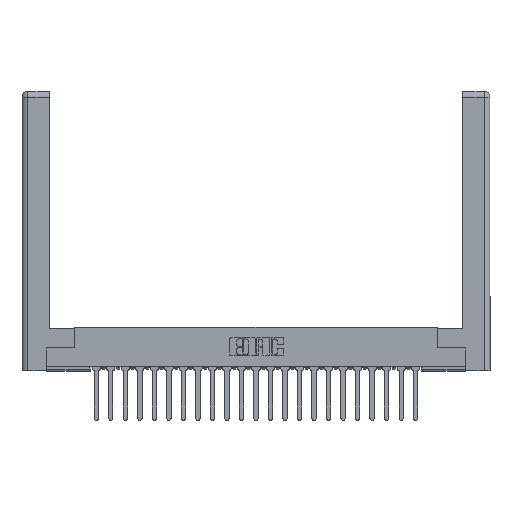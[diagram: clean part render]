
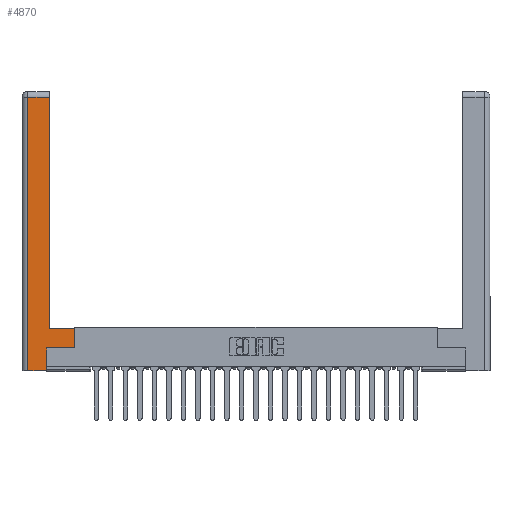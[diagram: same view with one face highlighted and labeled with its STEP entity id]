
A CAD part, top view. The second image highlights one B-rep face of the part: STEP entity #4870.
In plain terms, the highlighted planar face has unit normal (0, 0, 1).
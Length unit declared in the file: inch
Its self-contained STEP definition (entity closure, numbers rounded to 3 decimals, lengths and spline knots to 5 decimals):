
#6 = DIRECTION ( 'NONE',  ( 0., 1., 0. ) ) ;
#18 = EDGE_CURVE ( 'NONE', #4970, #5522, #1642, .T. ) ;
#577 = LINE ( 'NONE', #17559, #17094 ) ;
#739 = ORIENTED_EDGE ( 'NONE', *, *, #7062, .T. ) ;
#1168 = DIRECTION ( 'NONE',  ( 0., 0., -1. ) ) ;
#1177 = EDGE_CURVE ( 'NONE', #13833, #18348, #10896, .T. ) ;
#1642 = LINE ( 'NONE', #16851, #24171 ) ;
#1664 = DIRECTION ( 'NONE',  ( -1., 0., 0. ) ) ;
#2560 = EDGE_LOOP ( 'NONE', ( #3241, #9305, #17655, #739, #11428, #19648, #7668, #17305 ) ) ;
#3241 = ORIENTED_EDGE ( 'NONE', *, *, #19728, .T. ) ;
#3547 = PLANE ( 'NONE',  #6704 ) ;
#4024 = CARTESIAN_POINT ( 'NONE',  ( 0.0615, 2.94, 0. ) ) ;
#4086 = VECTOR ( 'NONE', #6, 39.37008 ) ;
#4566 = CARTESIAN_POINT ( 'NONE',  ( 0.295, 2.94, 0. ) ) ;
#4767 = EDGE_CURVE ( 'NONE', #21797, #19455, #18626, .T. ) ;
#4870 = ADVANCED_FACE ( 'NONE', ( #11147 ), #3547, .F. ) ;
#4970 = VERTEX_POINT ( 'NONE', #4024 ) ;
#5487 = CARTESIAN_POINT ( 'NONE',  ( 0.265, 0., 0. ) ) ;
#5522 = VERTEX_POINT ( 'NONE', #14090 ) ;
#5541 = VECTOR ( 'NONE', #15188, 39.37008 ) ;
#6074 = CARTESIAN_POINT ( 'NONE',  ( 0.0615, 2.94, 0. ) ) ;
#6196 = DIRECTION ( 'NONE',  ( -1., 0., 0. ) ) ;
#6300 = DIRECTION ( 'NONE',  ( 0., 1., 0. ) ) ;
#6704 = AXIS2_PLACEMENT_3D ( 'NONE', #16386, #1168, #1664 ) ;
#7062 = EDGE_CURVE ( 'NONE', #5522, #21797, #21164, .T. ) ;
#7386 = DIRECTION ( 'NONE',  ( 0., -1., 0. ) ) ;
#7668 = ORIENTED_EDGE ( 'NONE', *, *, #1177, .T. ) ;
#7795 = VECTOR ( 'NONE', #20074, 39.37008 ) ;
#8369 = EDGE_CURVE ( 'NONE', #19455, #13833, #577, .T. ) ;
#9305 = ORIENTED_EDGE ( 'NONE', *, *, #20843, .T. ) ;
#9650 = CARTESIAN_POINT ( 'NONE',  ( 0.565, 0.45, 0. ) ) ;
#10896 = LINE ( 'NONE', #18494, #4086 ) ;
#11147 = FACE_OUTER_BOUND ( 'NONE', #2560, .T. ) ;
#11428 = ORIENTED_EDGE ( 'NONE', *, *, #4767, .T. ) ;
#11572 = CARTESIAN_POINT ( 'NONE',  ( 0.295, 0.45, 0. ) ) ;
#13833 = VERTEX_POINT ( 'NONE', #22338 ) ;
#13887 = VECTOR ( 'NONE', #6300, 39.37008 ) ;
#14090 = CARTESIAN_POINT ( 'NONE',  ( 0.0615, 0., 0. ) ) ;
#14361 = VERTEX_POINT ( 'NONE', #11572 ) ;
#15188 = DIRECTION ( 'NONE',  ( 1., 0., 0. ) ) ;
#15413 = EDGE_CURVE ( 'NONE', #18348, #14361, #15847, .T. ) ;
#15535 = LINE ( 'NONE', #6074, #19091 ) ;
#15810 = DIRECTION ( 'NONE',  ( 1., 0., 0. ) ) ;
#15847 = LINE ( 'NONE', #23444, #7795 ) ;
#16216 = VERTEX_POINT ( 'NONE', #4566 ) ;
#16386 = CARTESIAN_POINT ( 'NONE',  ( 0., 0., 0. ) ) ;
#16851 = CARTESIAN_POINT ( 'NONE',  ( 0.0615, 0., 0. ) ) ;
#17094 = VECTOR ( 'NONE', #15810, 39.37008 ) ;
#17305 = ORIENTED_EDGE ( 'NONE', *, *, #15413, .T. ) ;
#17559 = CARTESIAN_POINT ( 'NONE',  ( 0.565, 0.245, 0. ) ) ;
#17629 = CARTESIAN_POINT ( 'NONE',  ( 0.295, 3., 0. ) ) ;
#17655 = ORIENTED_EDGE ( 'NONE', *, *, #18, .T. ) ;
#18348 = VERTEX_POINT ( 'NONE', #9650 ) ;
#18494 = CARTESIAN_POINT ( 'NONE',  ( 0.565, 0.45, 0. ) ) ;
#18626 = LINE ( 'NONE', #22105, #22977 ) ;
#19091 = VECTOR ( 'NONE', #6196, 39.37008 ) ;
#19455 = VERTEX_POINT ( 'NONE', #20147 ) ;
#19648 = ORIENTED_EDGE ( 'NONE', *, *, #8369, .T. ) ;
#19728 = EDGE_CURVE ( 'NONE', #14361, #16216, #20993, .T. ) ;
#20074 = DIRECTION ( 'NONE',  ( -1., 0., 0. ) ) ;
#20147 = CARTESIAN_POINT ( 'NONE',  ( 0.265, 0.245, 0. ) ) ;
#20843 = EDGE_CURVE ( 'NONE', #16216, #4970, #15535, .T. ) ;
#20993 = LINE ( 'NONE', #17629, #13887 ) ;
#21164 = LINE ( 'NONE', #5487, #5541 ) ;
#21274 = CARTESIAN_POINT ( 'NONE',  ( 0.265, 0., 0. ) ) ;
#21797 = VERTEX_POINT ( 'NONE', #21274 ) ;
#22105 = CARTESIAN_POINT ( 'NONE',  ( 0.265, 0.245, 0. ) ) ;
#22338 = CARTESIAN_POINT ( 'NONE',  ( 0.565, 0.245, 0. ) ) ;
#22977 = VECTOR ( 'NONE', #24372, 39.37008 ) ;
#23444 = CARTESIAN_POINT ( 'NONE',  ( 0.295, 0.45, 0. ) ) ;
#24171 = VECTOR ( 'NONE', #7386, 39.37008 ) ;
#24372 = DIRECTION ( 'NONE',  ( 0., 1., 0. ) ) ;
